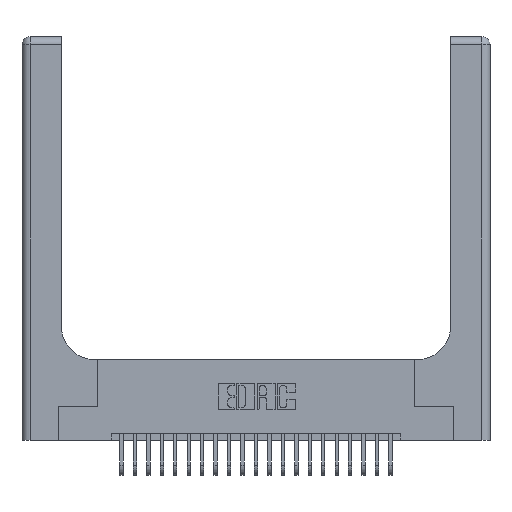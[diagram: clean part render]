
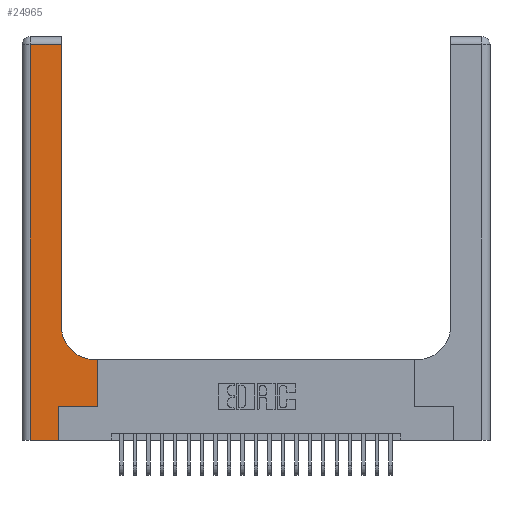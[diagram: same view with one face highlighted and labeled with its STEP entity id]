
A CAD part, top view. The second image highlights one B-rep face of the part: STEP entity #24965.
In plain terms, the highlighted planar face has unit normal (0, 0, 1).
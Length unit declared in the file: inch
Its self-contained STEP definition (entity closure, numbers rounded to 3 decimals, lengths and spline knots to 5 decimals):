
#26 = FACE_OUTER_BOUND ( 'NONE', #25183, .T. ) ;
#848 = CARTESIAN_POINT ( 'NONE',  ( 0., 3., 0.37 ) ) ;
#1013 = EDGE_CURVE ( 'NONE', #24297, #13559, #16931, .T. ) ;
#1839 = VERTEX_POINT ( 'NONE', #25614 ) ;
#1889 = EDGE_CURVE ( 'NONE', #1839, #11744, #13440, .T. ) ;
#2675 = VERTEX_POINT ( 'NONE', #9891 ) ;
#2885 = ORIENTED_EDGE ( 'NONE', *, *, #18292, .T. ) ;
#3384 = CARTESIAN_POINT ( 'NONE',  ( 0.06, 2.94, 0.37 ) ) ;
#3878 = AXIS2_PLACEMENT_3D ( 'NONE', #10820, #24973, #12880 ) ;
#4047 = CARTESIAN_POINT ( 'NONE',  ( 0.2915, 2.94, 0.37 ) ) ;
#4189 = ORIENTED_EDGE ( 'NONE', *, *, #22030, .T. ) ;
#4292 = CARTESIAN_POINT ( 'NONE',  ( 0., 2.94, 0.37 ) ) ;
#4729 = EDGE_CURVE ( 'NONE', #15825, #24297, #18640, .T. ) ;
#4784 = DIRECTION ( 'NONE',  ( 0., 1., 0. ) ) ;
#4909 = PLANE ( 'NONE',  #7283 ) ;
#6074 = ORIENTED_EDGE ( 'NONE', *, *, #4729, .T. ) ;
#6193 = CARTESIAN_POINT ( 'NONE',  ( 0.5415, 0.6, 0.37 ) ) ;
#7130 = LINE ( 'NONE', #23008, #26093 ) ;
#7283 = AXIS2_PLACEMENT_3D ( 'NONE', #848, #10983, #25129 ) ;
#7600 = DIRECTION ( 'NONE',  ( 0., 1., 0. ) ) ;
#8518 = ORIENTED_EDGE ( 'NONE', *, *, #1013, .T. ) ;
#8774 = CARTESIAN_POINT ( 'NONE',  ( 0.2915, 3., 0.37 ) ) ;
#8801 = CARTESIAN_POINT ( 'NONE',  ( 0.2915, 0.85, 0.37 ) ) ;
#8867 = DIRECTION ( 'NONE',  ( 0., -1., 0. ) ) ;
#9765 = ORIENTED_EDGE ( 'NONE', *, *, #10084, .T. ) ;
#9891 = CARTESIAN_POINT ( 'NONE',  ( 0.06, 0., 0.37 ) ) ;
#10084 = EDGE_CURVE ( 'NONE', #23993, #2675, #14146, .T. ) ;
#10809 = EDGE_CURVE ( 'NONE', #2675, #20519, #7130, .T. ) ;
#10820 = CARTESIAN_POINT ( 'NONE',  ( 0.5415, 0.85, 0.37 ) ) ;
#10906 = CARTESIAN_POINT ( 'NONE',  ( 0.06, 3., 0.37 ) ) ;
#10983 = DIRECTION ( 'NONE',  ( 0., 0., -1. ) ) ;
#11576 = VECTOR ( 'NONE', #24958, 39.37008 ) ;
#11744 = VERTEX_POINT ( 'NONE', #12277 ) ;
#12277 = CARTESIAN_POINT ( 'NONE',  ( 0.5585, 0.6, 0.37 ) ) ;
#12301 = VECTOR ( 'NONE', #4784, 39.37008 ) ;
#12880 = DIRECTION ( 'NONE',  ( 1., 0., 0. ) ) ;
#13114 = VECTOR ( 'NONE', #15207, 39.37008 ) ;
#13175 = CARTESIAN_POINT ( 'NONE',  ( 0.2915, 0.6, 0.37 ) ) ;
#13440 = LINE ( 'NONE', #19710, #23552 ) ;
#13521 = VECTOR ( 'NONE', #8867, 39.37008 ) ;
#13559 = VERTEX_POINT ( 'NONE', #4047 ) ;
#14146 = LINE ( 'NONE', #10906, #13521 ) ;
#14204 = EDGE_CURVE ( 'NONE', #13559, #23993, #18287, .T. ) ;
#14386 = LINE ( 'NONE', #13175, #13114 ) ;
#14594 = ORIENTED_EDGE ( 'NONE', *, *, #1889, .T. ) ;
#15173 = DIRECTION ( 'NONE',  ( 1., 0., 0. ) ) ;
#15207 = DIRECTION ( 'NONE',  ( -1., 0., 0. ) ) ;
#15825 = VERTEX_POINT ( 'NONE', #6193 ) ;
#16365 = DIRECTION ( 'NONE',  ( -1., 0., 0. ) ) ;
#16460 = ORIENTED_EDGE ( 'NONE', *, *, #10809, .T. ) ;
#16867 = CARTESIAN_POINT ( 'NONE',  ( 0.269, 0., 0.37 ) ) ;
#16931 = LINE ( 'NONE', #8774, #11576 ) ;
#17014 = LINE ( 'NONE', #16867, #12301 ) ;
#17714 = ORIENTED_EDGE ( 'NONE', *, *, #19461, .T. ) ;
#18287 = LINE ( 'NONE', #4292, #23679 ) ;
#18292 = EDGE_CURVE ( 'NONE', #23322, #1839, #21252, .T. ) ;
#18640 = CIRCLE ( 'NONE', #3878, 0.25 ) ;
#19461 = EDGE_CURVE ( 'NONE', #20519, #23322, #17014, .T. ) ;
#19710 = CARTESIAN_POINT ( 'NONE',  ( 0.5585, 0.25, 0.37 ) ) ;
#19786 = CARTESIAN_POINT ( 'NONE',  ( 0.269, 0., 0.37 ) ) ;
#20519 = VERTEX_POINT ( 'NONE', #19786 ) ;
#20560 = ORIENTED_EDGE ( 'NONE', *, *, #14204, .T. ) ;
#20994 = CARTESIAN_POINT ( 'NONE',  ( 0.269, 0.25, 0.37 ) ) ;
#21062 = DIRECTION ( 'NONE',  ( 1., 0., 0. ) ) ;
#21252 = LINE ( 'NONE', #25218, #22523 ) ;
#22030 = EDGE_CURVE ( 'NONE', #11744, #15825, #14386, .T. ) ;
#22523 = VECTOR ( 'NONE', #15173, 39.37008 ) ;
#23008 = CARTESIAN_POINT ( 'NONE',  ( 0., 0., 0.37 ) ) ;
#23322 = VERTEX_POINT ( 'NONE', #20994 ) ;
#23552 = VECTOR ( 'NONE', #7600, 39.37008 ) ;
#23679 = VECTOR ( 'NONE', #16365, 39.37008 ) ;
#23993 = VERTEX_POINT ( 'NONE', #3384 ) ;
#24297 = VERTEX_POINT ( 'NONE', #8801 ) ;
#24958 = DIRECTION ( 'NONE',  ( 0., 1., 0. ) ) ;
#24965 = ADVANCED_FACE ( 'NONE', ( #26 ), #4909, .F. ) ;
#24973 = DIRECTION ( 'NONE',  ( 0., 0., -1. ) ) ;
#25129 = DIRECTION ( 'NONE',  ( -1., 0., 0. ) ) ;
#25183 = EDGE_LOOP ( 'NONE', ( #8518, #20560, #9765, #16460, #17714, #2885, #14594, #4189, #6074 ) ) ;
#25218 = CARTESIAN_POINT ( 'NONE',  ( 0.269, 0.25, 0.37 ) ) ;
#25614 = CARTESIAN_POINT ( 'NONE',  ( 0.5585, 0.25, 0.37 ) ) ;
#26093 = VECTOR ( 'NONE', #21062, 39.37008 ) ;
